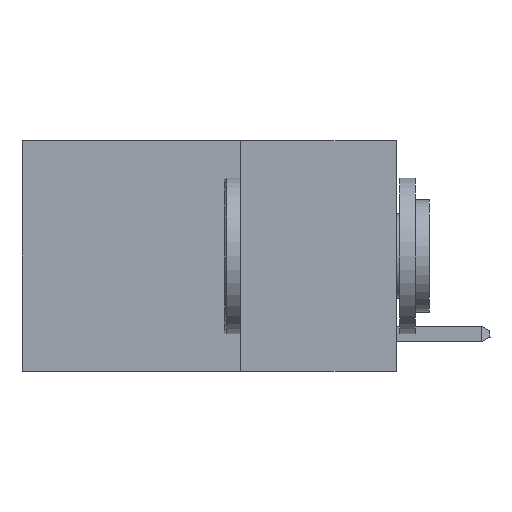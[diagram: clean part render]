
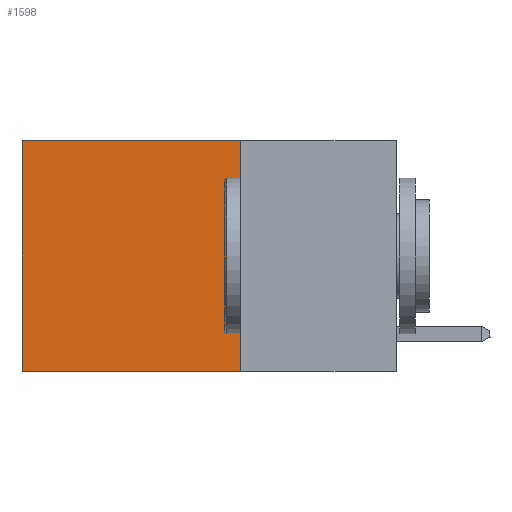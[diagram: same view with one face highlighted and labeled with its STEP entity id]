
A CAD part, left-side view. The second image highlights one B-rep face of the part: STEP entity #1598.
In plain terms, the highlighted planar face has unit normal (-1, 0, 0).
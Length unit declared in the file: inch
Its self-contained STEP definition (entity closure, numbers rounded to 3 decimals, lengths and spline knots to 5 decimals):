
#21 = CARTESIAN_POINT ( 'NONE',  ( 0.2625, 0.25, 0. ) ) ;
#96 = LINE ( 'NONE', #3465, #645 ) ;
#432 = ORIENTED_EDGE ( 'NONE', *, *, #9269, .T. ) ;
#636 = EDGE_CURVE ( 'NONE', #10181, #1668, #3721, .T. ) ;
#645 = VECTOR ( 'NONE', #5970, 39.37008 ) ;
#652 = LINE ( 'NONE', #2466, #6967 ) ;
#705 = DIRECTION ( 'NONE',  ( 0., 1., 0. ) ) ;
#717 = DIRECTION ( 'NONE',  ( 0., 0., -1. ) ) ;
#831 = CARTESIAN_POINT ( 'NONE',  ( 0.2625, 0.6, 0. ) ) ;
#886 = VECTOR ( 'NONE', #4762, 39.37008 ) ;
#896 = DIRECTION ( 'NONE',  ( 0., 0., -1. ) ) ;
#947 = DIRECTION ( 'NONE',  ( 1., 0., 0. ) ) ;
#1417 = CARTESIAN_POINT ( 'NONE',  ( 0.2625, 0.25, 0. ) ) ;
#1586 = AXIS2_PLACEMENT_3D ( 'NONE', #21, #947, #896 ) ;
#1598 = ADVANCED_FACE ( 'NONE', ( #2708 ), #6157, .F. ) ;
#1668 = VERTEX_POINT ( 'NONE', #7707 ) ;
#2160 = ORIENTED_EDGE ( 'NONE', *, *, #2662, .F. ) ;
#2466 = CARTESIAN_POINT ( 'NONE',  ( 0.2625, 0.25, 0. ) ) ;
#2662 = EDGE_CURVE ( 'NONE', #5078, #1668, #96, .T. ) ;
#2708 = FACE_OUTER_BOUND ( 'NONE', #8545, .T. ) ;
#3465 = CARTESIAN_POINT ( 'NONE',  ( 0.2625, 0.25, -0.37 ) ) ;
#3721 = LINE ( 'NONE', #8453, #5799 ) ;
#4762 = DIRECTION ( 'NONE',  ( 0., 0., -1. ) ) ;
#4929 = ORIENTED_EDGE ( 'NONE', *, *, #9094, .F. ) ;
#5078 = VERTEX_POINT ( 'NONE', #7855 ) ;
#5799 = VECTOR ( 'NONE', #717, 39.37008 ) ;
#5970 = DIRECTION ( 'NONE',  ( 0., 1., 0. ) ) ;
#6157 = PLANE ( 'NONE',  #1586 ) ;
#6465 = LINE ( 'NONE', #6519, #886 ) ;
#6519 = CARTESIAN_POINT ( 'NONE',  ( 0.2625, 0.25, 0. ) ) ;
#6967 = VECTOR ( 'NONE', #705, 39.37008 ) ;
#7707 = CARTESIAN_POINT ( 'NONE',  ( 0.2625, 0.6, -0.37 ) ) ;
#7855 = CARTESIAN_POINT ( 'NONE',  ( 0.2625, 0.25, -0.37 ) ) ;
#7866 = ORIENTED_EDGE ( 'NONE', *, *, #636, .T. ) ;
#8453 = CARTESIAN_POINT ( 'NONE',  ( 0.2625, 0.6, 0. ) ) ;
#8545 = EDGE_LOOP ( 'NONE', ( #7866, #2160, #4929, #432 ) ) ;
#9094 = EDGE_CURVE ( 'NONE', #9233, #5078, #6465, .T. ) ;
#9233 = VERTEX_POINT ( 'NONE', #1417 ) ;
#9269 = EDGE_CURVE ( 'NONE', #9233, #10181, #652, .T. ) ;
#10181 = VERTEX_POINT ( 'NONE', #831 ) ;
